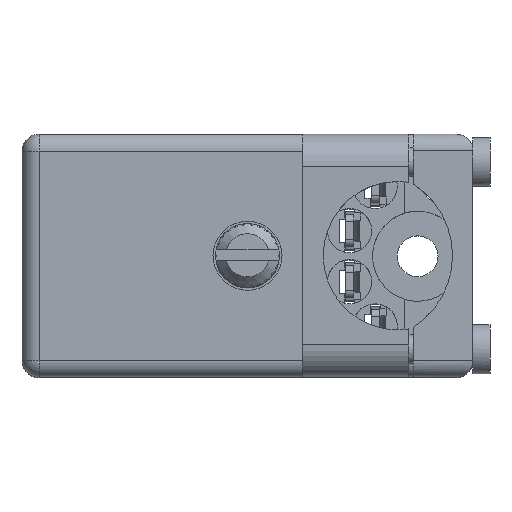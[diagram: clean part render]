
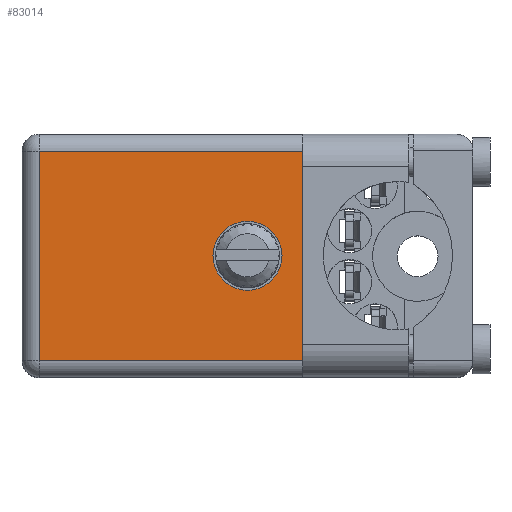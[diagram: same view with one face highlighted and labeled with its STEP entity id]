
A CAD part, top view. The second image highlights one B-rep face of the part: STEP entity #83014.
In plain terms, the highlighted face is planar.
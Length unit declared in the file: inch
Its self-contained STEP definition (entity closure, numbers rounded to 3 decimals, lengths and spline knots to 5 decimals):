
#2457 = DIRECTION ( 'NONE',  ( 0., 0., 1. ) ) ;
#2971 = VERTEX_POINT ( 'NONE', #69017 ) ;
#4970 = CARTESIAN_POINT ( 'NONE',  ( 0.05, 0.906, -0.05 ) ) ;
#6005 = ORIENTED_EDGE ( 'NONE', *, *, #137444, .T. ) ;
#6393 = VECTOR ( 'NONE', #156801, 39.37008 ) ;
#7325 = VECTOR ( 'NONE', #121987, 39.37008 ) ;
#8121 = ORIENTED_EDGE ( 'NONE', *, *, #157594, .F. ) ;
#8444 = CIRCLE ( 'NONE', #186477, 0.1015 ) ;
#8588 = VERTEX_POINT ( 'NONE', #132046 ) ;
#11520 = CARTESIAN_POINT ( 'NONE',  ( 1.15, 0.906, -0.665 ) ) ;
#11785 = CARTESIAN_POINT ( 'NONE',  ( 0.865, 0.906, -0.1125 ) ) ;
#16807 = CARTESIAN_POINT ( 'NONE',  ( 0., 0.906, -0.715 ) ) ;
#17456 = CARTESIAN_POINT ( 'NONE',  ( 0.865, 0.906, -0.6025 ) ) ;
#18168 = CARTESIAN_POINT ( 'NONE',  ( 1.15, 0.906, -0.1125 ) ) ;
#29062 = EDGE_CURVE ( 'NONE', #2971, #49226, #32592, .T. ) ;
#29856 = DIRECTION ( 'NONE',  ( 0., 0., -1. ) ) ;
#32592 = LINE ( 'NONE', #151748, #7325 ) ;
#33206 = DIRECTION ( 'NONE',  ( 0., 0., 1. ) ) ;
#39562 = CARTESIAN_POINT ( 'NONE',  ( 0., 0.906, -0.665 ) ) ;
#41699 = AXIS2_PLACEMENT_3D ( 'NONE', #16807, #134133, #2457 ) ;
#43567 = LINE ( 'NONE', #132954, #62333 ) ;
#44263 = LINE ( 'NONE', #134620, #63583 ) ;
#49226 = VERTEX_POINT ( 'NONE', #4970 ) ;
#51447 = LINE ( 'NONE', #126425, #147342 ) ;
#61303 = EDGE_LOOP ( 'NONE', ( #8121, #183046 ) ) ;
#62038 = CARTESIAN_POINT ( 'NONE',  ( 0.6625, 0.906, -0.3575 ) ) ;
#62333 = VECTOR ( 'NONE', #85011, 39.37008 ) ;
#63500 = ORIENTED_EDGE ( 'NONE', *, *, #177198, .T. ) ;
#63583 = VECTOR ( 'NONE', #29856, 39.37008 ) ;
#64149 = VERTEX_POINT ( 'NONE', #11520 ) ;
#65809 = DIRECTION ( 'NONE',  ( 0., 1., 0. ) ) ;
#68320 = EDGE_CURVE ( 'NONE', #123533, #86214, #43567, .T. ) ;
#69017 = CARTESIAN_POINT ( 'NONE',  ( 0.05, 0.906, -0.665 ) ) ;
#71292 = VECTOR ( 'NONE', #136403, 39.37008 ) ;
#77464 = CARTESIAN_POINT ( 'NONE',  ( 1.15, 0.906, -0.715 ) ) ;
#81833 = VERTEX_POINT ( 'NONE', #11785 ) ;
#82214 = DIRECTION ( 'NONE',  ( 1., 0., 0. ) ) ;
#83014 = ADVANCED_FACE ( 'NONE', ( #148539, #162967 ), #159173, .T. ) ;
#85011 = DIRECTION ( 'NONE',  ( 0., 0., 1. ) ) ;
#85589 = AXIS2_PLACEMENT_3D ( 'NONE', #62038, #65809, #33206 ) ;
#86214 = VERTEX_POINT ( 'NONE', #120215 ) ;
#87085 = ORIENTED_EDGE ( 'NONE', *, *, #125652, .T. ) ;
#89100 = DIRECTION ( 'NONE',  ( 0., 0., 1. ) ) ;
#94912 = VERTEX_POINT ( 'NONE', #17456 ) ;
#103213 = ORIENTED_EDGE ( 'NONE', *, *, #29062, .T. ) ;
#108415 = ORIENTED_EDGE ( 'NONE', *, *, #68320, .F. ) ;
#113399 = ORIENTED_EDGE ( 'NONE', *, *, #150141, .T. ) ;
#117865 = CARTESIAN_POINT ( 'NONE',  ( 0.6625, 0.906, -0.3575 ) ) ;
#117932 = LINE ( 'NONE', #77464, #141443 ) ;
#118347 = ORIENTED_EDGE ( 'NONE', *, *, #118507, .T. ) ;
#118507 = EDGE_CURVE ( 'NONE', #64149, #2971, #128910, .T. ) ;
#120215 = CARTESIAN_POINT ( 'NONE',  ( 1.15, 0.906, -0.05 ) ) ;
#121987 = DIRECTION ( 'NONE',  ( 0., 0., 1. ) ) ;
#123533 = VERTEX_POINT ( 'NONE', #18168 ) ;
#125652 = EDGE_CURVE ( 'NONE', #94912, #179045, #135464, .T. ) ;
#126425 = CARTESIAN_POINT ( 'NONE',  ( 1.15, 0.906, -0.05 ) ) ;
#128910 = LINE ( 'NONE', #39562, #6393 ) ;
#130370 = DIRECTION ( 'NONE',  ( 0., 1., 0. ) ) ;
#132046 = CARTESIAN_POINT ( 'NONE',  ( 0.6625, 0.906, -0.459 ) ) ;
#132954 = CARTESIAN_POINT ( 'NONE',  ( 1.15, 0.906, -0.715 ) ) ;
#134133 = DIRECTION ( 'NONE',  ( 0., 1., 0. ) ) ;
#134620 = CARTESIAN_POINT ( 'NONE',  ( 0.865, 0.906, -0.1125 ) ) ;
#135464 = LINE ( 'NONE', #166190, #71292 ) ;
#136396 = DIRECTION ( 'NONE',  ( -1., 0., 0. ) ) ;
#136403 = DIRECTION ( 'NONE',  ( 1., 0., 0. ) ) ;
#137444 = EDGE_CURVE ( 'NONE', #123533, #81833, #150819, .T. ) ;
#141443 = VECTOR ( 'NONE', #89100, 39.37008 ) ;
#145783 = ORIENTED_EDGE ( 'NONE', *, *, #181984, .F. ) ;
#146696 = VERTEX_POINT ( 'NONE', #160637 ) ;
#147031 = CARTESIAN_POINT ( 'NONE',  ( 0.865, 0.906, -0.1125 ) ) ;
#147342 = VECTOR ( 'NONE', #82214, 39.37008 ) ;
#148539 = FACE_OUTER_BOUND ( 'NONE', #168916, .T. ) ;
#150048 = CIRCLE ( 'NONE', #85589, 0.1015 ) ;
#150141 = EDGE_CURVE ( 'NONE', #81833, #94912, #44263, .T. ) ;
#150410 = EDGE_CURVE ( 'NONE', #8588, #146696, #8444, .T. ) ;
#150819 = LINE ( 'NONE', #147031, #185813 ) ;
#151748 = CARTESIAN_POINT ( 'NONE',  ( 0.05, 0.906, -0.715 ) ) ;
#156801 = DIRECTION ( 'NONE',  ( -1., 0., 0. ) ) ;
#157594 = EDGE_CURVE ( 'NONE', #146696, #8588, #150048, .T. ) ;
#159173 = PLANE ( 'NONE',  #41699 ) ;
#160637 = CARTESIAN_POINT ( 'NONE',  ( 0.6625, 0.906, -0.256 ) ) ;
#162967 = FACE_BOUND ( 'NONE', #61303, .T. ) ;
#166190 = CARTESIAN_POINT ( 'NONE',  ( 0.865, 0.906, -0.6025 ) ) ;
#168916 = EDGE_LOOP ( 'NONE', ( #103213, #63500, #108415, #6005, #113399, #87085, #145783, #118347 ) ) ;
#175541 = DIRECTION ( 'NONE',  ( 0., 0., 1. ) ) ;
#177198 = EDGE_CURVE ( 'NONE', #49226, #86214, #51447, .T. ) ;
#179045 = VERTEX_POINT ( 'NONE', #188514 ) ;
#181984 = EDGE_CURVE ( 'NONE', #64149, #179045, #117932, .T. ) ;
#183046 = ORIENTED_EDGE ( 'NONE', *, *, #150410, .F. ) ;
#185813 = VECTOR ( 'NONE', #136396, 39.37008 ) ;
#186477 = AXIS2_PLACEMENT_3D ( 'NONE', #117865, #130370, #175541 ) ;
#188514 = CARTESIAN_POINT ( 'NONE',  ( 1.15, 0.906, -0.6025 ) ) ;
